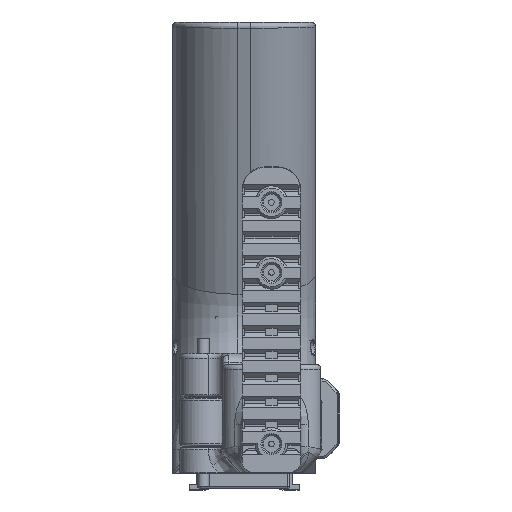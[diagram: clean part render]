
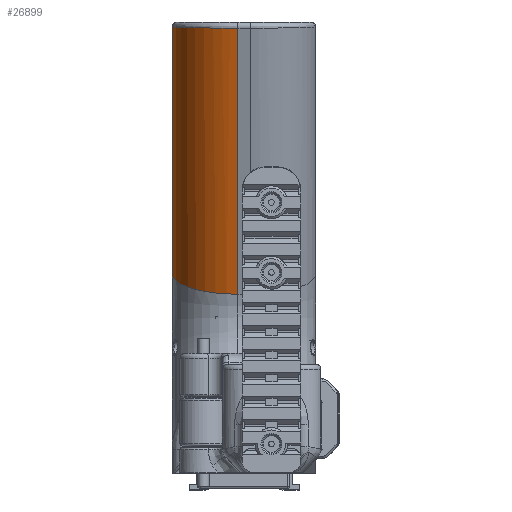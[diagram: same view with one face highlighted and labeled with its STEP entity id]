
A CAD part, left-side view. The second image highlights one B-rep face of the part: STEP entity #26899.
In plain terms, the highlighted cylindrical face has radius 14 mm (diameter 28 mm), a partial arc.
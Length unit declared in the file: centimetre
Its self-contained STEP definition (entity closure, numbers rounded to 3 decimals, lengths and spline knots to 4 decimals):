
#512=ELLIPSE($,#28963,1.4623,1.4);
#2595=LINE($,#43811,#4623);
#2597=LINE($,#43815,#4625);
#4623=VECTOR($,#33892,5.9599);
#4625=VECTOR($,#33896,5.5376);
#6937=FACE_OUTER_BOUND($,#8655,.T.);
#8655=EDGE_LOOP($,(#20824,#20825,#20826,#20827));
#10061=CIRCLE($,#28992,1.4);
#11951=VERTEX_POINT($,#43542);
#11952=VERTEX_POINT($,#43587);
#12002=VERTEX_POINT($,#43810);
#12003=VERTEX_POINT($,#43814);
#15070=EDGE_CURVE($,#11951,#11952,#512,.T.);
#15127=EDGE_CURVE($,#12002,#11952,#2595,.T.);
#15129=EDGE_CURVE($,#11951,#12003,#2597,.T.);
#15130=EDGE_CURVE($,#12002,#12003,#10061,.T.);
#20824=ORIENTED_EDGE($,*,*,#15070,.F.);
#20825=ORIENTED_EDGE($,*,*,#15129,.T.);
#20826=ORIENTED_EDGE($,*,*,#15130,.F.);
#20827=ORIENTED_EDGE($,*,*,#15127,.T.);
#25941=CYLINDRICAL_SURFACE($,#28991,1.4);
#26899=ADVANCED_FACE($,(#6937),#25941,.T.);
#28963=AXIS2_PLACEMENT_3D($,#43589,#33808,#33809);
#28991=AXIS2_PLACEMENT_3D($,#43813,#33894,#33895);
#28992=AXIS2_PLACEMENT_3D($,#43816,#33897,#33898);
#33808=DIRECTION('center_axis',(-0.021,0.,
1.));
#33809=DIRECTION('ref_axis',(-1.,0.,-0.021));
#33892=DIRECTION($,(-0.309,0.,0.951));
#33894=DIRECTION('center_axis',(-0.309,0.,0.951));
#33895=DIRECTION('ref_axis',(-0.672,0.707,-0.219));
#33896=DIRECTION($,(0.309,0.,-0.951));
#33897=DIRECTION('center_axis',(0.309,0.,-0.951));
#33898=DIRECTION('ref_axis',(-0.951,0.,-0.309));
#43542=CARTESIAN_POINT('',(-7.2435,11.505,5.5075));
#43587=CARTESIAN_POINT('',(-8.7055,10.105,5.4766));
#43589=CARTESIAN_POINT('Origin',(-7.2435,10.105,5.5075));
#43810=CARTESIAN_POINT('',(-6.8637,10.105,-0.1917));
#43811=CARTESIAN_POINT($,(-6.786,10.105,-0.4308));
#43813=CARTESIAN_POINT('Origin',(-5.8254,10.105,1.1431));
#43814=CARTESIAN_POINT('',(-5.5323,11.505,0.241));
#43815=CARTESIAN_POINT($,(-5.8254,11.505,1.1431));
#43816=CARTESIAN_POINT('Origin',(-5.5323,10.105,0.241));
